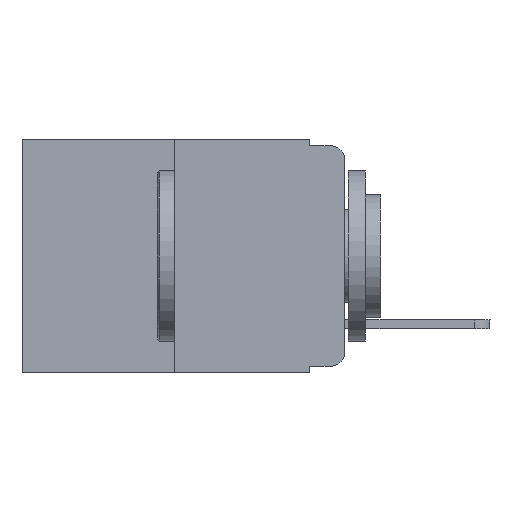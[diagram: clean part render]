
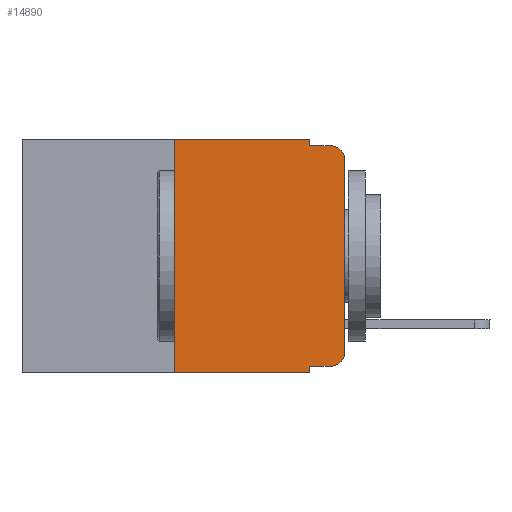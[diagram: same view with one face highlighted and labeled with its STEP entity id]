
A CAD part, left-side view. The second image highlights one B-rep face of the part: STEP entity #14890.
In plain terms, the highlighted planar face has unit normal (-1, 0, 0).
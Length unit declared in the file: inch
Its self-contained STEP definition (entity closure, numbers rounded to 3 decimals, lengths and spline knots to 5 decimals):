
#204 = CIRCLE ( 'NONE', #17570, 0.02 ) ;
#233 = CARTESIAN_POINT ( 'NONE',  ( 0., 0.051, -0.01 ) ) ;
#1083 = VERTEX_POINT ( 'NONE', #10478 ) ;
#1712 = DIRECTION ( 'NONE',  ( 0., -1., 0. ) ) ;
#1884 = EDGE_CURVE ( 'NONE', #2018, #8859, #2655, .T. ) ;
#1908 = EDGE_CURVE ( 'NONE', #15381, #8623, #17330, .T. ) ;
#2002 = DIRECTION ( 'NONE',  ( -1., 0., 0. ) ) ;
#2018 = VERTEX_POINT ( 'NONE', #14708 ) ;
#2155 = VECTOR ( 'NONE', #14822, 39.37008 ) ;
#2603 = CARTESIAN_POINT ( 'NONE',  ( 0., 0.473, -0.343 ) ) ;
#2655 = CIRCLE ( 'NONE', #21508, 0.02 ) ;
#2714 = VERTEX_POINT ( 'NONE', #3575 ) ;
#2837 = DIRECTION ( 'NONE',  ( 0., -1., 0. ) ) ;
#2934 = ORIENTED_EDGE ( 'NONE', *, *, #1908, .F. ) ;
#3099 = LINE ( 'NONE', #15192, #8024 ) ;
#3575 = CARTESIAN_POINT ( 'NONE',  ( 0., 0.051, -0.343 ) ) ;
#4590 = DIRECTION ( 'NONE',  ( 1., 0., 0. ) ) ;
#5043 = DIRECTION ( 'NONE',  ( 0., 0., -1. ) ) ;
#5084 = LINE ( 'NONE', #6441, #14511 ) ;
#5507 = ORIENTED_EDGE ( 'NONE', *, *, #1884, .T. ) ;
#5539 = DIRECTION ( 'NONE',  ( -1., 0., 0. ) ) ;
#5991 = ORIENTED_EDGE ( 'NONE', *, *, #22000, .F. ) ;
#6441 = CARTESIAN_POINT ( 'NONE',  ( 0., 0.051, -0.01 ) ) ;
#6714 = VERTEX_POINT ( 'NONE', #11413 ) ;
#6957 = LINE ( 'NONE', #18967, #7798 ) ;
#7798 = VECTOR ( 'NONE', #5043, 39.37008 ) ;
#7870 = ORIENTED_EDGE ( 'NONE', *, *, #14777, .T. ) ;
#8024 = VECTOR ( 'NONE', #10743, 39.37008 ) ;
#8191 = ORIENTED_EDGE ( 'NONE', *, *, #19010, .T. ) ;
#8395 = VERTEX_POINT ( 'NONE', #233 ) ;
#8623 = VERTEX_POINT ( 'NONE', #8668 ) ;
#8666 = CARTESIAN_POINT ( 'NONE',  ( 0., 0., 0. ) ) ;
#8668 = CARTESIAN_POINT ( 'NONE',  ( 0., 0.051, 0. ) ) ;
#8859 = VERTEX_POINT ( 'NONE', #16149 ) ;
#8878 = CARTESIAN_POINT ( 'NONE',  ( 0., 0.02, -0.313 ) ) ;
#9509 = EDGE_CURVE ( 'NONE', #6714, #15092, #20845, .T. ) ;
#10333 = ORIENTED_EDGE ( 'NONE', *, *, #21087, .F. ) ;
#10439 = CARTESIAN_POINT ( 'NONE',  ( 0., 0.02, -0.333 ) ) ;
#10478 = CARTESIAN_POINT ( 'NONE',  ( 0., 0.25, -0.343 ) ) ;
#10569 = ORIENTED_EDGE ( 'NONE', *, *, #9509, .T. ) ;
#10743 = DIRECTION ( 'NONE',  ( 0., 0., -1. ) ) ;
#11171 = LINE ( 'NONE', #2603, #2155 ) ;
#11413 = CARTESIAN_POINT ( 'NONE',  ( 0., 0.051, -0.333 ) ) ;
#12316 = CARTESIAN_POINT ( 'NONE',  ( 0., 0.25, 0. ) ) ;
#12859 = LINE ( 'NONE', #19766, #18957 ) ;
#12953 = DIRECTION ( 'NONE',  ( 0., 0., -1. ) ) ;
#13165 = EDGE_CURVE ( 'NONE', #1083, #15381, #12859, .T. ) ;
#13590 = AXIS2_PLACEMENT_3D ( 'NONE', #19747, #4590, #12953 ) ;
#14260 = ORIENTED_EDGE ( 'NONE', *, *, #14600, .T. ) ;
#14511 = VECTOR ( 'NONE', #2837, 39.37008 ) ;
#14600 = EDGE_CURVE ( 'NONE', #22343, #2018, #20671, .T. ) ;
#14670 = VECTOR ( 'NONE', #1712, 39.37008 ) ;
#14674 = VECTOR ( 'NONE', #19084, 39.37008 ) ;
#14708 = CARTESIAN_POINT ( 'NONE',  ( 0., 0., -0.03 ) ) ;
#14777 = EDGE_CURVE ( 'NONE', #15092, #22343, #204, .T. ) ;
#14822 = DIRECTION ( 'NONE',  ( 0., -1., 0. ) ) ;
#14890 = ADVANCED_FACE ( 'NONE', ( #21562 ), #21677, .F. ) ;
#15092 = VERTEX_POINT ( 'NONE', #10439 ) ;
#15192 = CARTESIAN_POINT ( 'NONE',  ( 0., 0.051, 0. ) ) ;
#15381 = VERTEX_POINT ( 'NONE', #12316 ) ;
#15634 = DIRECTION ( 'NONE',  ( 0., 0., -1. ) ) ;
#16149 = CARTESIAN_POINT ( 'NONE',  ( 0., 0.02, -0.01 ) ) ;
#16656 = EDGE_CURVE ( 'NONE', #8623, #8395, #6957, .T. ) ;
#17088 = ORIENTED_EDGE ( 'NONE', *, *, #16656, .F. ) ;
#17242 = DIRECTION ( 'NONE',  ( 0., -1., 0. ) ) ;
#17330 = LINE ( 'NONE', #17547, #14670 ) ;
#17547 = CARTESIAN_POINT ( 'NONE',  ( 0., 0.473, 0. ) ) ;
#17570 = AXIS2_PLACEMENT_3D ( 'NONE', #8878, #2002, #17728 ) ;
#17583 = DIRECTION ( 'NONE',  ( 0., 0., 1. ) ) ;
#17728 = DIRECTION ( 'NONE',  ( 0., 0., -1. ) ) ;
#18170 = EDGE_LOOP ( 'NONE', ( #14260, #5507, #10333, #17088, #2934, #20867, #8191, #5991, #10569, #7870 ) ) ;
#18926 = CARTESIAN_POINT ( 'NONE',  ( 0., 0.051, -0.333 ) ) ;
#18957 = VECTOR ( 'NONE', #17583, 39.37008 ) ;
#18967 = CARTESIAN_POINT ( 'NONE',  ( 0., 0.051, 0. ) ) ;
#19010 = EDGE_CURVE ( 'NONE', #1083, #2714, #11171, .T. ) ;
#19084 = DIRECTION ( 'NONE',  ( 0., 0., 1. ) ) ;
#19231 = VECTOR ( 'NONE', #17242, 39.37008 ) ;
#19747 = CARTESIAN_POINT ( 'NONE',  ( 0., 0.473, 0. ) ) ;
#19766 = CARTESIAN_POINT ( 'NONE',  ( 0., 0.25, 0. ) ) ;
#20265 = CARTESIAN_POINT ( 'NONE',  ( 0., 0., -0.313 ) ) ;
#20671 = LINE ( 'NONE', #8666, #14674 ) ;
#20845 = LINE ( 'NONE', #18926, #19231 ) ;
#20867 = ORIENTED_EDGE ( 'NONE', *, *, #13165, .F. ) ;
#21047 = CARTESIAN_POINT ( 'NONE',  ( 0., 0.02, -0.03 ) ) ;
#21087 = EDGE_CURVE ( 'NONE', #8395, #8859, #5084, .T. ) ;
#21508 = AXIS2_PLACEMENT_3D ( 'NONE', #21047, #5539, #15634 ) ;
#21562 = FACE_OUTER_BOUND ( 'NONE', #18170, .T. ) ;
#21677 = PLANE ( 'NONE',  #13590 ) ;
#22000 = EDGE_CURVE ( 'NONE', #6714, #2714, #3099, .T. ) ;
#22343 = VERTEX_POINT ( 'NONE', #20265 ) ;
